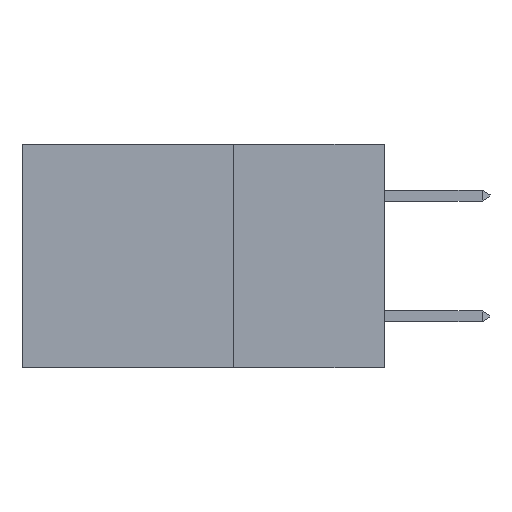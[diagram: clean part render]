
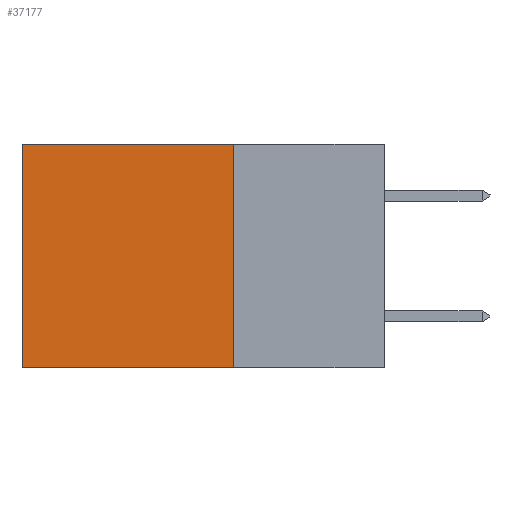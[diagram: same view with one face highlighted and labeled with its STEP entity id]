
A CAD part, left-side view. The second image highlights one B-rep face of the part: STEP entity #37177.
In plain terms, the highlighted planar face has unit normal (-1, 0, 0).
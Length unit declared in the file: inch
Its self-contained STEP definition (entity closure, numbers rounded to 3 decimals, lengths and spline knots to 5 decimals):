
#710 = LINE ( 'NONE', #26722, #32769 ) ;
#3653 = EDGE_LOOP ( 'NONE', ( #36651, #36364, #27914, #9624 ) ) ;
#3940 = EDGE_CURVE ( 'NONE', #34402, #40619, #710, .T. ) ;
#4815 = EDGE_CURVE ( 'NONE', #29668, #34402, #37266, .T. ) ;
#4945 = CARTESIAN_POINT ( 'NONE',  ( 0.2875, 0.25, -0.37 ) ) ;
#8805 = CARTESIAN_POINT ( 'NONE',  ( 0.2875, 0.25, 0. ) ) ;
#9624 = ORIENTED_EDGE ( 'NONE', *, *, #4815, .T. ) ;
#10126 = DIRECTION ( 'NONE',  ( 0., 0., -1. ) ) ;
#11380 = CARTESIAN_POINT ( 'NONE',  ( 0.2875, 0.6, 0. ) ) ;
#11453 = DIRECTION ( 'NONE',  ( 0., 1., 0. ) ) ;
#12024 = DIRECTION ( 'NONE',  ( 1., 0., 0. ) ) ;
#12185 = LINE ( 'NONE', #32396, #36627 ) ;
#16141 = EDGE_CURVE ( 'NONE', #29693, #40619, #31390, .T. ) ;
#17741 = CARTESIAN_POINT ( 'NONE',  ( 0.2875, 0.25, 0. ) ) ;
#18848 = EDGE_CURVE ( 'NONE', #29668, #29693, #12185, .T. ) ;
#19274 = CARTESIAN_POINT ( 'NONE',  ( 0.2875, 0.25, -0.37 ) ) ;
#20328 = VECTOR ( 'NONE', #27374, 39.37008 ) ;
#22910 = VECTOR ( 'NONE', #11453, 39.37008 ) ;
#24144 = CARTESIAN_POINT ( 'NONE',  ( 0.2875, 0.25, 0. ) ) ;
#26722 = CARTESIAN_POINT ( 'NONE',  ( 0.2875, 0.6, 0. ) ) ;
#27374 = DIRECTION ( 'NONE',  ( 0., 1., 0. ) ) ;
#27914 = ORIENTED_EDGE ( 'NONE', *, *, #18848, .F. ) ;
#27938 = PLANE ( 'NONE',  #29553 ) ;
#29553 = AXIS2_PLACEMENT_3D ( 'NONE', #8805, #12024, #34319 ) ;
#29668 = VERTEX_POINT ( 'NONE', #17741 ) ;
#29693 = VERTEX_POINT ( 'NONE', #4945 ) ;
#29942 = DIRECTION ( 'NONE',  ( 0., 0., -1. ) ) ;
#31390 = LINE ( 'NONE', #19274, #22910 ) ;
#32396 = CARTESIAN_POINT ( 'NONE',  ( 0.2875, 0.25, 0. ) ) ;
#32769 = VECTOR ( 'NONE', #29942, 39.37008 ) ;
#34251 = FACE_OUTER_BOUND ( 'NONE', #3653, .T. ) ;
#34319 = DIRECTION ( 'NONE',  ( 0., 0., -1. ) ) ;
#34402 = VERTEX_POINT ( 'NONE', #11380 ) ;
#36364 = ORIENTED_EDGE ( 'NONE', *, *, #16141, .F. ) ;
#36627 = VECTOR ( 'NONE', #10126, 39.37008 ) ;
#36651 = ORIENTED_EDGE ( 'NONE', *, *, #3940, .T. ) ;
#37177 = ADVANCED_FACE ( 'NONE', ( #34251 ), #27938, .F. ) ;
#37266 = LINE ( 'NONE', #24144, #20328 ) ;
#39708 = CARTESIAN_POINT ( 'NONE',  ( 0.2875, 0.6, -0.37 ) ) ;
#40619 = VERTEX_POINT ( 'NONE', #39708 ) ;
